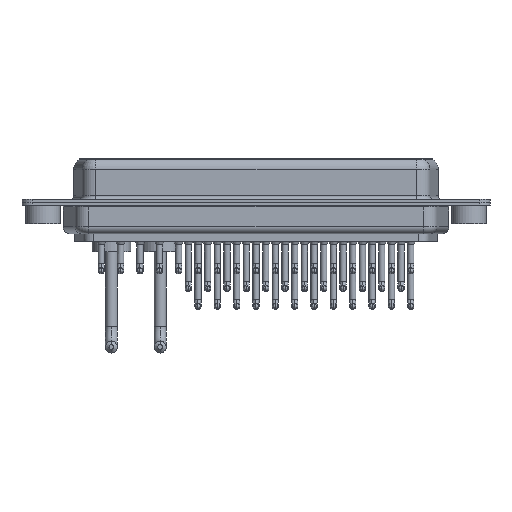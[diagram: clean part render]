
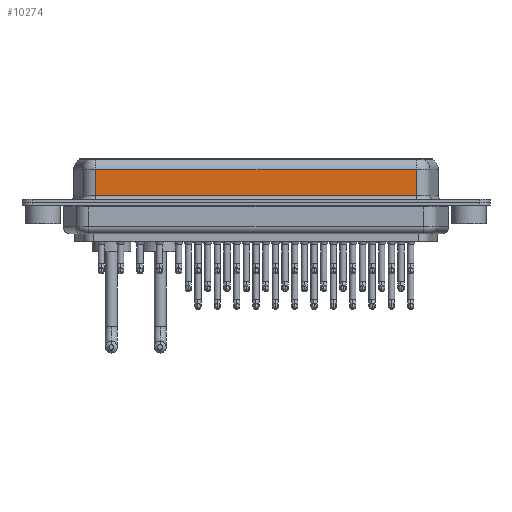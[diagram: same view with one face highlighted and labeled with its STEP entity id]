
A CAD part, front view. The second image highlights one B-rep face of the part: STEP entity #10274.
In plain terms, the highlighted planar face has unit normal (0, -1, 0).
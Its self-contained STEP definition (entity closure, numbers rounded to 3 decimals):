
#1269 = LINE ( 'NONE', #25636, #7996 ) ;
#2734 = ORIENTED_EDGE ( 'NONE', *, *, #8072, .F. ) ;
#3601 = VERTEX_POINT ( 'NONE', #9928 ) ;
#4045 = VECTOR ( 'NONE', #30050, 1000. ) ;
#4457 = PLANE ( 'NONE',  #12157 ) ;
#5900 = DIRECTION ( 'NONE',  ( 0., 0., -1. ) ) ;
#7316 = DIRECTION ( 'NONE',  ( 0., 0., -1. ) ) ;
#7996 = VECTOR ( 'NONE', #5900, 1000. ) ;
#8072 = EDGE_CURVE ( 'NONE', #17120, #24219, #25212, .T. ) ;
#8778 = EDGE_CURVE ( 'NONE', #12844, #24219, #32330, .T. ) ;
#9647 = DIRECTION ( 'NONE',  ( 1., 0., 0. ) ) ;
#9733 = DIRECTION ( 'NONE',  ( 0., 0., 1. ) ) ;
#9928 = CARTESIAN_POINT ( 'NONE',  ( 7.59, -5.375, 4.65 ) ) ;
#10274 = ADVANCED_FACE ( 'NONE', ( #21575 ), #4457, .F. ) ;
#12088 = ORIENTED_EDGE ( 'NONE', *, *, #31579, .T. ) ;
#12157 = AXIS2_PLACEMENT_3D ( 'NONE', #19132, #29118, #9733 ) ;
#12289 = EDGE_CURVE ( 'NONE', #3601, #12844, #1269, .T. ) ;
#12581 = CARTESIAN_POINT ( 'NONE',  ( 53.41, -5.375, 6.4 ) ) ;
#12656 = CARTESIAN_POINT ( 'NONE',  ( 53.41, -5.375, 4.65 ) ) ;
#12844 = VERTEX_POINT ( 'NONE', #24088 ) ;
#16189 = CARTESIAN_POINT ( 'NONE',  ( 53.41, -5.375, 0.9 ) ) ;
#16737 = CARTESIAN_POINT ( 'NONE',  ( 53.41, -5.375, 0.9 ) ) ;
#17120 = VERTEX_POINT ( 'NONE', #28444 ) ;
#19132 = CARTESIAN_POINT ( 'NONE',  ( 53.41, -5.375, 6.4 ) ) ;
#20703 = LINE ( 'NONE', #12656, #4045 ) ;
#20970 = VECTOR ( 'NONE', #9647, 1000. ) ;
#21575 = FACE_OUTER_BOUND ( 'NONE', #28858, .T. ) ;
#23066 = VECTOR ( 'NONE', #7316, 1000. ) ;
#24088 = CARTESIAN_POINT ( 'NONE',  ( 7.59, -5.375, 0.9 ) ) ;
#24219 = VERTEX_POINT ( 'NONE', #16189 ) ;
#25212 = LINE ( 'NONE', #12581, #23066 ) ;
#25636 = CARTESIAN_POINT ( 'NONE',  ( 7.59, -5.375, 6.4 ) ) ;
#26500 = ORIENTED_EDGE ( 'NONE', *, *, #12289, .T. ) ;
#28444 = CARTESIAN_POINT ( 'NONE',  ( 53.41, -5.375, 4.65 ) ) ;
#28858 = EDGE_LOOP ( 'NONE', ( #2734, #12088, #26500, #29922 ) ) ;
#29118 = DIRECTION ( 'NONE',  ( 0., 1., 0. ) ) ;
#29922 = ORIENTED_EDGE ( 'NONE', *, *, #8778, .T. ) ;
#30050 = DIRECTION ( 'NONE',  ( -1., 0., 0. ) ) ;
#31579 = EDGE_CURVE ( 'NONE', #17120, #3601, #20703, .T. ) ;
#32330 = LINE ( 'NONE', #16737, #20970 ) ;
